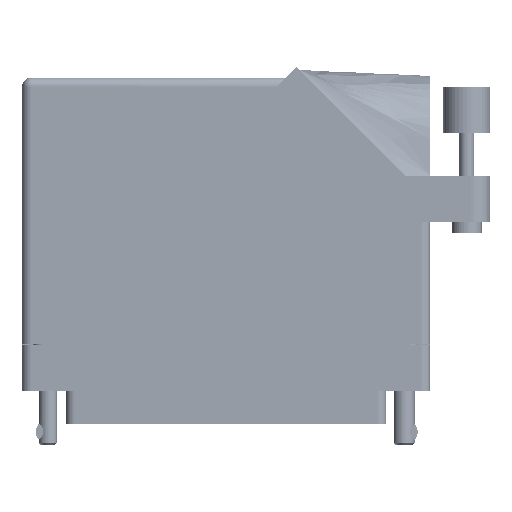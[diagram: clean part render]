
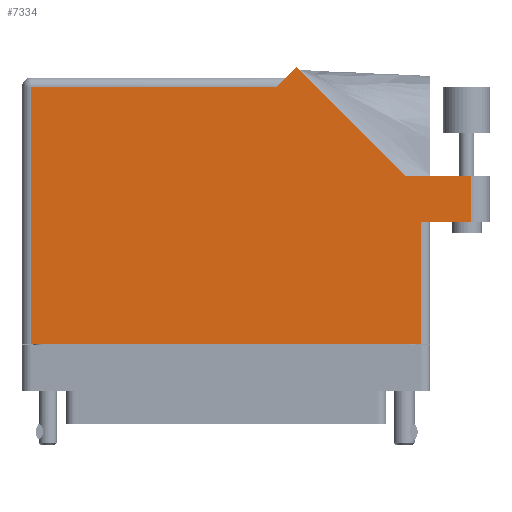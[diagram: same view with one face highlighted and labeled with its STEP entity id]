
A CAD part, front view. The second image highlights one B-rep face of the part: STEP entity #7334.
In plain terms, the highlighted face is planar.
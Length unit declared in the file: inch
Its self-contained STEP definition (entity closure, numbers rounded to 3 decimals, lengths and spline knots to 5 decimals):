
#303 = CARTESIAN_POINT ( 'NONE',  ( 1.634, 0.715, 0.617 ) ) ;
#446 = EDGE_CURVE ( 'NONE', #53394, #83620, #21931, .T. ) ;
#1222 = FACE_OUTER_BOUND ( 'NONE', #58113, .T. ) ;
#1279 = DIRECTION ( 'NONE',  ( -0.707, -0.707, 0. ) ) ;
#1629 = CARTESIAN_POINT ( 'NONE',  ( 1.19342, 1.022, 0.617 ) ) ;
#2460 = LINE ( 'NONE', #59593, #45042 ) ;
#2555 = EDGE_CURVE ( 'NONE', #5748, #53394, #2460, .T. ) ;
#3979 = LINE ( 'NONE', #24064, #27319 ) ;
#4694 = VECTOR ( 'NONE', #16290, 39.37008 ) ;
#5334 = CARTESIAN_POINT ( 'NONE',  ( 1.634, 1.022, 0.617 ) ) ;
#5370 = ORIENTED_EDGE ( 'NONE', *, *, #63234, .T. ) ;
#5748 = VERTEX_POINT ( 'NONE', #5334 ) ;
#5854 = CARTESIAN_POINT ( 'NONE',  ( -1.297, -0.1, 0.617 ) ) ;
#7164 = DIRECTION ( 'NONE',  ( -1., 0., 0. ) ) ;
#7334 = ADVANCED_FACE ( 'NONE', ( #1222 ), #37182, .F. ) ;
#11048 = CARTESIAN_POINT ( 'NONE',  ( 1.359, 0.715, 0.617 ) ) ;
#13421 = LINE ( 'NONE', #11048, #26570 ) ;
#13480 = CARTESIAN_POINT ( 'NONE',  ( 1.19342, 1.022, 0.617 ) ) ;
#15893 = DIRECTION ( 'NONE',  ( 0., 1., 0. ) ) ;
#16290 = DIRECTION ( 'NONE',  ( -0.707, 0.707, 0. ) ) ;
#17870 = ORIENTED_EDGE ( 'NONE', *, *, #19996, .T. ) ;
#18625 = EDGE_CURVE ( 'NONE', #65206, #5748, #72375, .T. ) ;
#19996 = EDGE_CURVE ( 'NONE', #72056, #45586, #43191, .T. ) ;
#20671 = DIRECTION ( 'NONE',  ( 0., 1., 0. ) ) ;
#21931 = LINE ( 'NONE', #1629, #4694 ) ;
#22427 = ORIENTED_EDGE ( 'NONE', *, *, #61100, .T. ) ;
#23614 = DIRECTION ( 'NONE',  ( 0., -1., 0. ) ) ;
#24064 = CARTESIAN_POINT ( 'NONE',  ( -1.359, -0.1, 0.617 ) ) ;
#24165 = CARTESIAN_POINT ( 'NONE',  ( -1.359, 1.675, 0.617 ) ) ;
#25016 = DIRECTION ( 'NONE',  ( 0., 0., -1. ) ) ;
#26570 = VECTOR ( 'NONE', #63189, 39.37008 ) ;
#26816 = CARTESIAN_POINT ( 'NONE',  ( 1.297, 0.715, 0.617 ) ) ;
#27319 = VECTOR ( 'NONE', #28854, 39.37008 ) ;
#27747 = CARTESIAN_POINT ( 'NONE',  ( 1.297, 0.715, 0.617 ) ) ;
#27973 = VECTOR ( 'NONE', #20671, 39.37008 ) ;
#28453 = LINE ( 'NONE', #56704, #77139 ) ;
#28854 = DIRECTION ( 'NONE',  ( 1., 0., 0. ) ) ;
#29110 = EDGE_CURVE ( 'NONE', #45339, #56340, #47831, .T. ) ;
#31721 = ORIENTED_EDGE ( 'NONE', *, *, #29110, .T. ) ;
#37182 = PLANE ( 'NONE',  #73409 ) ;
#39834 = VECTOR ( 'NONE', #1279, 39.37008 ) ;
#40705 = CARTESIAN_POINT ( 'NONE',  ( 0.46971, 1.74571, 0.617 ) ) ;
#43191 = LINE ( 'NONE', #27747, #27973 ) ;
#45042 = VECTOR ( 'NONE', #7164, 39.37008 ) ;
#45339 = VERTEX_POINT ( 'NONE', #76540 ) ;
#45586 = VERTEX_POINT ( 'NONE', #26816 ) ;
#47407 = CARTESIAN_POINT ( 'NONE',  ( 0.399, 1.675, 0.617 ) ) ;
#47831 = LINE ( 'NONE', #55710, #57017 ) ;
#47990 = ORIENTED_EDGE ( 'NONE', *, *, #70799, .T. ) ;
#49501 = VECTOR ( 'NONE', #15893, 39.37008 ) ;
#51217 = ORIENTED_EDGE ( 'NONE', *, *, #18625, .T. ) ;
#53394 = VERTEX_POINT ( 'NONE', #13480 ) ;
#55710 = CARTESIAN_POINT ( 'NONE',  ( -1.297, -0.1, 0.617 ) ) ;
#56340 = VERTEX_POINT ( 'NONE', #5854 ) ;
#56426 = ORIENTED_EDGE ( 'NONE', *, *, #68176, .T. ) ;
#56704 = CARTESIAN_POINT ( 'NONE',  ( -1.359, 1.613, 0.617 ) ) ;
#57017 = VECTOR ( 'NONE', #23614, 39.37008 ) ;
#58113 = EDGE_LOOP ( 'NONE', ( #56426, #51217, #70844, #72857, #22427, #47990, #31721, #5370, #17870 ) ) ;
#59593 = CARTESIAN_POINT ( 'NONE',  ( 1.759, 1.022, 0.617 ) ) ;
#61100 = EDGE_CURVE ( 'NONE', #83620, #68451, #63207, .T. ) ;
#61551 = CARTESIAN_POINT ( 'NONE',  ( 1.634, 1.022, 0.617 ) ) ;
#62440 = CARTESIAN_POINT ( 'NONE',  ( 0.337, 1.613, 0.617 ) ) ;
#63186 = DIRECTION ( 'NONE',  ( -1., 0., 0. ) ) ;
#63189 = DIRECTION ( 'NONE',  ( 1., 0., 0. ) ) ;
#63207 = LINE ( 'NONE', #47407, #39834 ) ;
#63234 = EDGE_CURVE ( 'NONE', #56340, #72056, #3979, .T. ) ;
#65206 = VERTEX_POINT ( 'NONE', #303 ) ;
#68176 = EDGE_CURVE ( 'NONE', #45586, #65206, #13421, .T. ) ;
#68451 = VERTEX_POINT ( 'NONE', #62440 ) ;
#70421 = DIRECTION ( 'NONE',  ( -1., 0., 0. ) ) ;
#70799 = EDGE_CURVE ( 'NONE', #68451, #45339, #28453, .T. ) ;
#70844 = ORIENTED_EDGE ( 'NONE', *, *, #2555, .T. ) ;
#72056 = VERTEX_POINT ( 'NONE', #73412 ) ;
#72375 = LINE ( 'NONE', #61551, #49501 ) ;
#72857 = ORIENTED_EDGE ( 'NONE', *, *, #446, .T. ) ;
#73409 = AXIS2_PLACEMENT_3D ( 'NONE', #24165, #25016, #70421 ) ;
#73412 = CARTESIAN_POINT ( 'NONE',  ( 1.297, -0.1, 0.617 ) ) ;
#76540 = CARTESIAN_POINT ( 'NONE',  ( -1.297, 1.613, 0.617 ) ) ;
#77139 = VECTOR ( 'NONE', #63186, 39.37008 ) ;
#83620 = VERTEX_POINT ( 'NONE', #40705 ) ;
